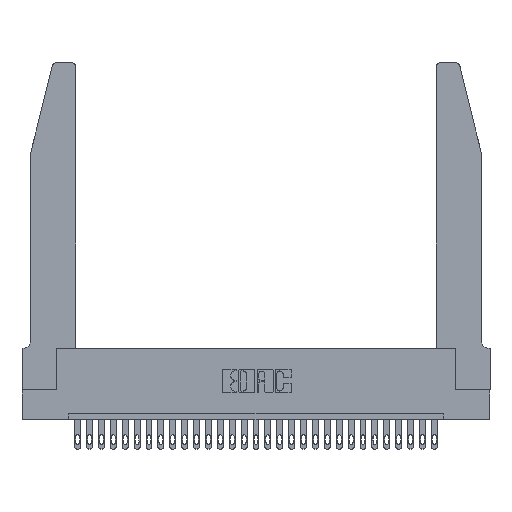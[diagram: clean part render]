
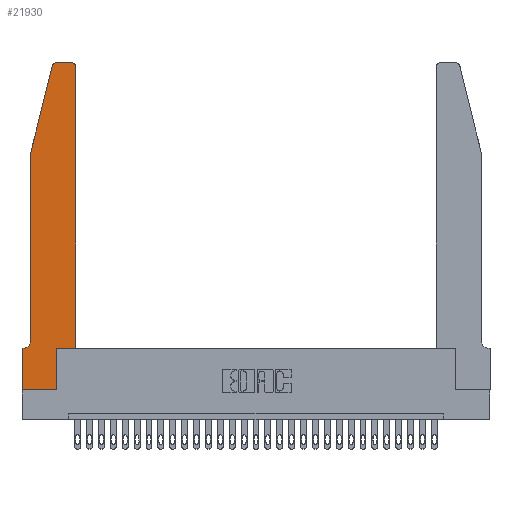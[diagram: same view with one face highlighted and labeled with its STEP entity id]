
A CAD part, top view. The second image highlights one B-rep face of the part: STEP entity #21930.
In plain terms, the highlighted planar face has unit normal (0, 0, 1).
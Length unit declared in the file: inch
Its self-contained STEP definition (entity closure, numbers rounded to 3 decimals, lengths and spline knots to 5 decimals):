
#2207 = CARTESIAN_POINT ( 'NONE',  ( 0.284, 2.72, 0.37 ) ) ;
#3017 = PLANE ( 'NONE',  #15889 ) ;
#3906 = ORIENTED_EDGE ( 'NONE', *, *, #4837, .T. ) ;
#4374 = CARTESIAN_POINT ( 'NONE',  ( 0.0755, 2., 0.37 ) ) ;
#4476 = DIRECTION ( 'NONE',  ( 0., 0., 1. ) ) ;
#4506 = DIRECTION ( 'NONE',  ( -1., 0., 0. ) ) ;
#4718 = EDGE_CURVE ( 'NONE', #19324, #28732, #22808, .T. ) ;
#4823 = CIRCLE ( 'NONE', #7401, 0.03 ) ;
#4837 = EDGE_CURVE ( 'NONE', #26816, #19324, #8876, .T. ) ;
#4947 = CARTESIAN_POINT ( 'NONE',  ( 0., 0., 0.37 ) ) ;
#5434 = LINE ( 'NONE', #23377, #18587 ) ;
#5576 = DIRECTION ( 'NONE',  ( 0., 0., -1. ) ) ;
#5632 = VERTEX_POINT ( 'NONE', #8860 ) ;
#5901 = CARTESIAN_POINT ( 'NONE',  ( 0., 0.35, 0.37 ) ) ;
#6174 = LINE ( 'NONE', #20046, #26126 ) ;
#6221 = CIRCLE ( 'NONE', #26579, 0.03 ) ;
#6538 = CARTESIAN_POINT ( 'NONE',  ( 0.4505, 2.72, 0.37 ) ) ;
#6679 = VECTOR ( 'NONE', #23874, 39.37008 ) ;
#6695 = CARTESIAN_POINT ( 'NONE',  ( 0.0055, 0.35, 0.37 ) ) ;
#6760 = DIRECTION ( 'NONE',  ( 1., 0., 0. ) ) ;
#7401 = AXIS2_PLACEMENT_3D ( 'NONE', #16005, #18308, #28045 ) ;
#7534 = CARTESIAN_POINT ( 'NONE',  ( 0., 0.35, 0.37 ) ) ;
#7780 = VERTEX_POINT ( 'NONE', #22253 ) ;
#7965 = VECTOR ( 'NONE', #4506, 39.37008 ) ;
#8137 = CARTESIAN_POINT ( 'NONE',  ( 0.0055, 0.42, 0.37 ) ) ;
#8738 = DIRECTION ( 'NONE',  ( 0., 1., 0. ) ) ;
#8767 = EDGE_CURVE ( 'NONE', #22201, #19940, #5434, .T. ) ;
#8860 = CARTESIAN_POINT ( 'NONE',  ( 0.25487, 2.72718, 0.37 ) ) ;
#8876 = LINE ( 'NONE', #11643, #26337 ) ;
#9173 = CARTESIAN_POINT ( 'NONE',  ( 0.0755, 2., 0.37 ) ) ;
#9197 = VERTEX_POINT ( 'NONE', #4374 ) ;
#10703 = CARTESIAN_POINT ( 'NONE',  ( 0.284, 2.75, 0.37 ) ) ;
#10716 = DIRECTION ( 'NONE',  ( 0., 1., 0. ) ) ;
#11108 = EDGE_CURVE ( 'NONE', #25280, #5632, #6221, .T. ) ;
#11441 = LINE ( 'NONE', #26521, #17824 ) ;
#11470 = CIRCLE ( 'NONE', #19013, 0.07 ) ;
#11643 = CARTESIAN_POINT ( 'NONE',  ( 0.4505, 0.35, 0.37 ) ) ;
#12034 = ORIENTED_EDGE ( 'NONE', *, *, #14002, .T. ) ;
#12169 = ORIENTED_EDGE ( 'NONE', *, *, #4718, .T. ) ;
#12472 = VECTOR ( 'NONE', #8738, 39.37008 ) ;
#12819 = DIRECTION ( 'NONE',  ( -1., 0., 0. ) ) ;
#13220 = ORIENTED_EDGE ( 'NONE', *, *, #25425, .T. ) ;
#13261 = EDGE_LOOP ( 'NONE', ( #22332, #25576, #13220, #24987, #21185, #23605, #23216, #26762, #12034, #3906, #12169, #15849 ) ) ;
#13560 = DIRECTION ( 'NONE',  ( -0.239, -0.971, 0. ) ) ;
#13869 = LINE ( 'NONE', #26141, #7965 ) ;
#13924 = EDGE_CURVE ( 'NONE', #26835, #22201, #11470, .T. ) ;
#14002 = EDGE_CURVE ( 'NONE', #27271, #26816, #11441, .T. ) ;
#14716 = EDGE_CURVE ( 'NONE', #7780, #25280, #13869, .T. ) ;
#15622 = CARTESIAN_POINT ( 'NONE',  ( 0.4505, 0.35, 0.37 ) ) ;
#15730 = DIRECTION ( 'NONE',  ( 0., 0., 1. ) ) ;
#15849 = ORIENTED_EDGE ( 'NONE', *, *, #18888, .T. ) ;
#15889 = AXIS2_PLACEMENT_3D ( 'NONE', #5901, #15730, #22927 ) ;
#16005 = CARTESIAN_POINT ( 'NONE',  ( 0.4205, 2.72, 0.37 ) ) ;
#16340 = CARTESIAN_POINT ( 'NONE',  ( 0.2865, 0.35, 0.37 ) ) ;
#17560 = EDGE_CURVE ( 'NONE', #9197, #26835, #26629, .T. ) ;
#17824 = VECTOR ( 'NONE', #10716, 39.37008 ) ;
#18308 = DIRECTION ( 'NONE',  ( 0., 0., 1. ) ) ;
#18587 = VECTOR ( 'NONE', #12819, 39.37008 ) ;
#18888 = EDGE_CURVE ( 'NONE', #28732, #7780, #4823, .T. ) ;
#19013 = AXIS2_PLACEMENT_3D ( 'NONE', #8137, #5576, #24094 ) ;
#19324 = VERTEX_POINT ( 'NONE', #15622 ) ;
#19448 = LINE ( 'NONE', #9173, #24065 ) ;
#19940 = VERTEX_POINT ( 'NONE', #7534 ) ;
#19969 = EDGE_CURVE ( 'NONE', #19940, #28859, #6174, .T. ) ;
#20046 = CARTESIAN_POINT ( 'NONE',  ( 0., 0., 0.37 ) ) ;
#20493 = DIRECTION ( 'NONE',  ( 1., 0., 0. ) ) ;
#21185 = ORIENTED_EDGE ( 'NONE', *, *, #13924, .T. ) ;
#21758 = VECTOR ( 'NONE', #22444, 39.37008 ) ;
#21930 = ADVANCED_FACE ( 'NONE', ( #23574 ), #3017, .T. ) ;
#22196 = DIRECTION ( 'NONE',  ( 0., -1., 0. ) ) ;
#22201 = VERTEX_POINT ( 'NONE', #6695 ) ;
#22253 = CARTESIAN_POINT ( 'NONE',  ( 0.4205, 2.75, 0.37 ) ) ;
#22332 = ORIENTED_EDGE ( 'NONE', *, *, #14716, .T. ) ;
#22444 = DIRECTION ( 'NONE',  ( 1., 0., 0. ) ) ;
#22808 = LINE ( 'NONE', #29442, #12472 ) ;
#22927 = DIRECTION ( 'NONE',  ( 1., 0., 0. ) ) ;
#23216 = ORIENTED_EDGE ( 'NONE', *, *, #19969, .T. ) ;
#23377 = CARTESIAN_POINT ( 'NONE',  ( 0.0755, 0.35, 0.37 ) ) ;
#23553 = CARTESIAN_POINT ( 'NONE',  ( 0.0755, 0.42, 0.37 ) ) ;
#23574 = FACE_OUTER_BOUND ( 'NONE', #13261, .T. ) ;
#23605 = ORIENTED_EDGE ( 'NONE', *, *, #8767, .T. ) ;
#23777 = CARTESIAN_POINT ( 'NONE',  ( 0.0755, 2., 0.37 ) ) ;
#23874 = DIRECTION ( 'NONE',  ( 0., -1., 0. ) ) ;
#24065 = VECTOR ( 'NONE', #13560, 39.37008 ) ;
#24094 = DIRECTION ( 'NONE',  ( -1., 0., 0. ) ) ;
#24987 = ORIENTED_EDGE ( 'NONE', *, *, #17560, .T. ) ;
#25280 = VERTEX_POINT ( 'NONE', #10703 ) ;
#25425 = EDGE_CURVE ( 'NONE', #5632, #9197, #19448, .T. ) ;
#25576 = ORIENTED_EDGE ( 'NONE', *, *, #11108, .T. ) ;
#26126 = VECTOR ( 'NONE', #22196, 39.37008 ) ;
#26141 = CARTESIAN_POINT ( 'NONE',  ( 0.2605, 2.75, 0.37 ) ) ;
#26337 = VECTOR ( 'NONE', #20493, 39.37008 ) ;
#26521 = CARTESIAN_POINT ( 'NONE',  ( 0.2865, 0.35, 0.37 ) ) ;
#26579 = AXIS2_PLACEMENT_3D ( 'NONE', #2207, #4476, #6760 ) ;
#26629 = LINE ( 'NONE', #23777, #6679 ) ;
#26724 = LINE ( 'NONE', #27093, #21758 ) ;
#26762 = ORIENTED_EDGE ( 'NONE', *, *, #28033, .T. ) ;
#26816 = VERTEX_POINT ( 'NONE', #16340 ) ;
#26835 = VERTEX_POINT ( 'NONE', #23553 ) ;
#27093 = CARTESIAN_POINT ( 'NONE',  ( 0., 0., 0.37 ) ) ;
#27271 = VERTEX_POINT ( 'NONE', #28331 ) ;
#28033 = EDGE_CURVE ( 'NONE', #28859, #27271, #26724, .T. ) ;
#28045 = DIRECTION ( 'NONE',  ( 1., 0., 0. ) ) ;
#28331 = CARTESIAN_POINT ( 'NONE',  ( 0.2865, 0., 0.37 ) ) ;
#28732 = VERTEX_POINT ( 'NONE', #6538 ) ;
#28859 = VERTEX_POINT ( 'NONE', #4947 ) ;
#29442 = CARTESIAN_POINT ( 'NONE',  ( 0.4505, 0.35, 0.37 ) ) ;
